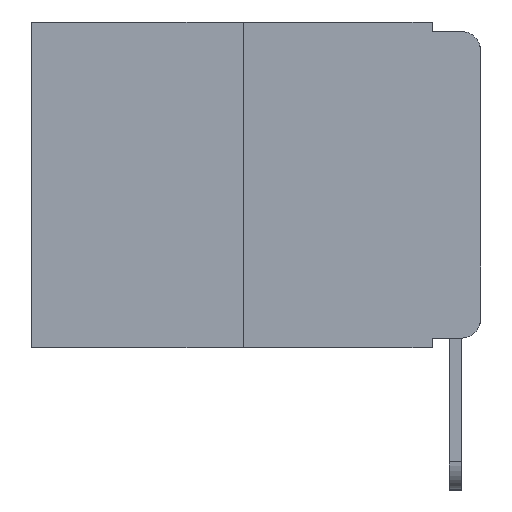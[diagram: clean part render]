
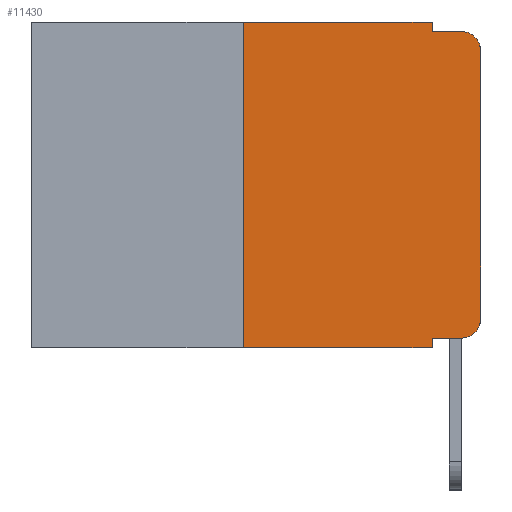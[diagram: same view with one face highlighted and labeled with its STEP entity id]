
A CAD part, left-side view. The second image highlights one B-rep face of the part: STEP entity #11430.
In plain terms, the highlighted planar face has unit normal (-1, 0, 0).
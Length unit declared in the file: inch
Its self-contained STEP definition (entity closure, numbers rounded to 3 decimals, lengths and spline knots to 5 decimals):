
#137 = CARTESIAN_POINT ( 'NONE',  ( 0., 0.02, -0.333 ) ) ;
#326 = CARTESIAN_POINT ( 'NONE',  ( 0., 0.02, -0.03 ) ) ;
#356 = CARTESIAN_POINT ( 'NONE',  ( 0., 0., -0.313 ) ) ;
#817 = DIRECTION ( 'NONE',  ( 0., -1., 0. ) ) ;
#919 = EDGE_CURVE ( 'NONE', #11818, #6668, #8535, .T. ) ;
#1069 = VECTOR ( 'NONE', #11693, 39.37008 ) ;
#1338 = CARTESIAN_POINT ( 'NONE',  ( 0., 0.051, -0.333 ) ) ;
#1375 = DIRECTION ( 'NONE',  ( 0., 0., -1. ) ) ;
#1604 = CIRCLE ( 'NONE', #1995, 0.02 ) ;
#1735 = CARTESIAN_POINT ( 'NONE',  ( 0., 0., 0. ) ) ;
#1995 = AXIS2_PLACEMENT_3D ( 'NONE', #8275, #2516, #9218 ) ;
#2029 = DIRECTION ( 'NONE',  ( 0., 0., -1. ) ) ;
#2262 = DIRECTION ( 'NONE',  ( 0., 0., 1. ) ) ;
#2318 = EDGE_CURVE ( 'NONE', #6799, #11818, #11394, .T. ) ;
#2384 = CARTESIAN_POINT ( 'NONE',  ( 0., 0.473, -0.343 ) ) ;
#2516 = DIRECTION ( 'NONE',  ( -1., 0., 0. ) ) ;
#2763 = DIRECTION ( 'NONE',  ( 0., 0., 1. ) ) ;
#3255 = VERTEX_POINT ( 'NONE', #9497 ) ;
#3319 = ORIENTED_EDGE ( 'NONE', *, *, #3913, .F. ) ;
#3711 = CARTESIAN_POINT ( 'NONE',  ( 0., 0.051, 0. ) ) ;
#3762 = CARTESIAN_POINT ( 'NONE',  ( 0., 0.051, -0.01 ) ) ;
#3848 = ORIENTED_EDGE ( 'NONE', *, *, #2318, .F. ) ;
#3913 = EDGE_CURVE ( 'NONE', #10028, #6799, #12062, .T. ) ;
#3925 = EDGE_CURVE ( 'NONE', #11364, #4734, #4911, .T. ) ;
#4019 = LINE ( 'NONE', #1735, #10908 ) ;
#4255 = ORIENTED_EDGE ( 'NONE', *, *, #919, .F. ) ;
#4482 = EDGE_LOOP ( 'NONE', ( #7697, #4787, #4255, #3848, #3319, #12217, #6529, #8428, #9436, #10686 ) ) ;
#4734 = VERTEX_POINT ( 'NONE', #137 ) ;
#4787 = ORIENTED_EDGE ( 'NONE', *, *, #10386, .T. ) ;
#4911 = LINE ( 'NONE', #1338, #7107 ) ;
#5388 = LINE ( 'NONE', #6060, #10345 ) ;
#5827 = CARTESIAN_POINT ( 'NONE',  ( 0., 0.051, -0.333 ) ) ;
#5851 = EDGE_CURVE ( 'NONE', #4734, #9174, #1604, .T. ) ;
#5938 = CARTESIAN_POINT ( 'NONE',  ( 0., 0.473, 0. ) ) ;
#6060 = CARTESIAN_POINT ( 'NONE',  ( 0., 0.051, 0. ) ) ;
#6126 = CARTESIAN_POINT ( 'NONE',  ( 0., 0.051, -0.01 ) ) ;
#6257 = VERTEX_POINT ( 'NONE', #12386 ) ;
#6525 = FACE_OUTER_BOUND ( 'NONE', #4482, .T. ) ;
#6529 = ORIENTED_EDGE ( 'NONE', *, *, #9786, .T. ) ;
#6668 = VERTEX_POINT ( 'NONE', #8338 ) ;
#6799 = VERTEX_POINT ( 'NONE', #3711 ) ;
#6999 = VECTOR ( 'NONE', #10047, 39.37008 ) ;
#7107 = VECTOR ( 'NONE', #817, 39.37008 ) ;
#7221 = DIRECTION ( 'NONE',  ( -1., 0., 0. ) ) ;
#7399 = VECTOR ( 'NONE', #12170, 39.37008 ) ;
#7461 = VERTEX_POINT ( 'NONE', #11984 ) ;
#7697 = ORIENTED_EDGE ( 'NONE', *, *, #10613, .T. ) ;
#7817 = DIRECTION ( 'NONE',  ( 1., 0., 0. ) ) ;
#8039 = CARTESIAN_POINT ( 'NONE',  ( 0., 0.25, 0. ) ) ;
#8275 = CARTESIAN_POINT ( 'NONE',  ( 0., 0.02, -0.313 ) ) ;
#8329 = VECTOR ( 'NONE', #9830, 39.37008 ) ;
#8338 = CARTESIAN_POINT ( 'NONE',  ( 0., 0.02, -0.01 ) ) ;
#8428 = ORIENTED_EDGE ( 'NONE', *, *, #10219, .F. ) ;
#8535 = LINE ( 'NONE', #6126, #1069 ) ;
#8602 = CARTESIAN_POINT ( 'NONE',  ( 0., 0.25, 0. ) ) ;
#8794 = VECTOR ( 'NONE', #2262, 39.37008 ) ;
#8907 = CIRCLE ( 'NONE', #12044, 0.02 ) ;
#9000 = EDGE_CURVE ( 'NONE', #7461, #10028, #11546, .T. ) ;
#9174 = VERTEX_POINT ( 'NONE', #356 ) ;
#9218 = DIRECTION ( 'NONE',  ( 0., 0., -1. ) ) ;
#9436 = ORIENTED_EDGE ( 'NONE', *, *, #3925, .T. ) ;
#9497 = CARTESIAN_POINT ( 'NONE',  ( 0., 0.051, -0.343 ) ) ;
#9654 = PLANE ( 'NONE',  #11751 ) ;
#9786 = EDGE_CURVE ( 'NONE', #7461, #3255, #11954, .T. ) ;
#9807 = CARTESIAN_POINT ( 'NONE',  ( 0., 0.051, 0. ) ) ;
#9830 = DIRECTION ( 'NONE',  ( 0., 0., -1. ) ) ;
#10028 = VERTEX_POINT ( 'NONE', #8602 ) ;
#10047 = DIRECTION ( 'NONE',  ( 0., -1., 0. ) ) ;
#10219 = EDGE_CURVE ( 'NONE', #11364, #3255, #5388, .T. ) ;
#10272 = CARTESIAN_POINT ( 'NONE',  ( 0., 0.473, 0. ) ) ;
#10345 = VECTOR ( 'NONE', #11637, 39.37008 ) ;
#10386 = EDGE_CURVE ( 'NONE', #6257, #6668, #8907, .T. ) ;
#10613 = EDGE_CURVE ( 'NONE', #9174, #6257, #4019, .T. ) ;
#10686 = ORIENTED_EDGE ( 'NONE', *, *, #5851, .T. ) ;
#10908 = VECTOR ( 'NONE', #2763, 39.37008 ) ;
#11364 = VERTEX_POINT ( 'NONE', #5827 ) ;
#11394 = LINE ( 'NONE', #9807, #8329 ) ;
#11430 = ADVANCED_FACE ( 'NONE', ( #6525 ), #9654, .F. ) ;
#11546 = LINE ( 'NONE', #8039, #8794 ) ;
#11637 = DIRECTION ( 'NONE',  ( 0., 0., -1. ) ) ;
#11693 = DIRECTION ( 'NONE',  ( 0., -1., 0. ) ) ;
#11751 = AXIS2_PLACEMENT_3D ( 'NONE', #5938, #7817, #2029 ) ;
#11818 = VERTEX_POINT ( 'NONE', #3762 ) ;
#11954 = LINE ( 'NONE', #2384, #6999 ) ;
#11984 = CARTESIAN_POINT ( 'NONE',  ( 0., 0.25, -0.343 ) ) ;
#12044 = AXIS2_PLACEMENT_3D ( 'NONE', #326, #7221, #1375 ) ;
#12062 = LINE ( 'NONE', #10272, #7399 ) ;
#12170 = DIRECTION ( 'NONE',  ( 0., -1., 0. ) ) ;
#12217 = ORIENTED_EDGE ( 'NONE', *, *, #9000, .F. ) ;
#12386 = CARTESIAN_POINT ( 'NONE',  ( 0., 0., -0.03 ) ) ;
